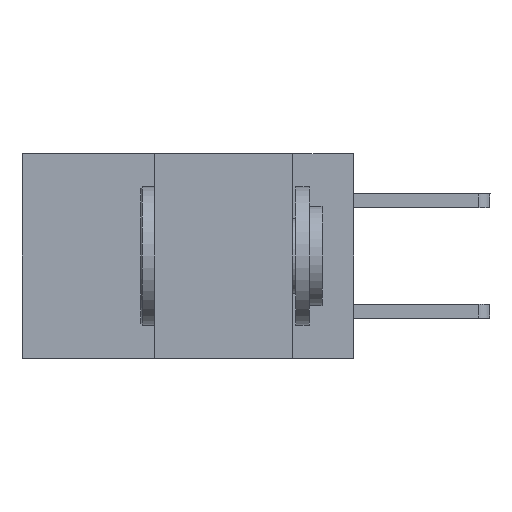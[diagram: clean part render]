
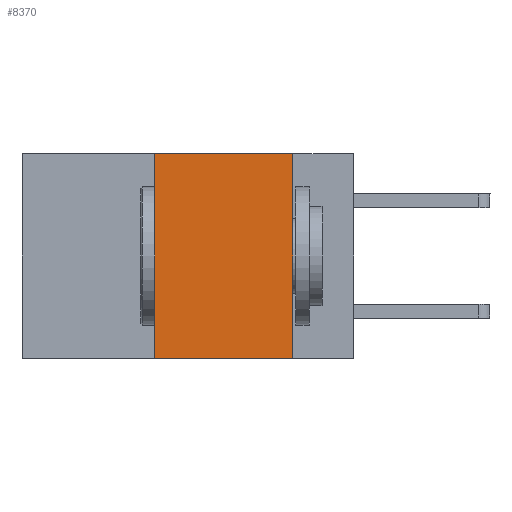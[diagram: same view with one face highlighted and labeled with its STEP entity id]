
A CAD part, left-side view. The second image highlights one B-rep face of the part: STEP entity #8370.
In plain terms, the highlighted planar face has unit normal (-1, 0, 0).
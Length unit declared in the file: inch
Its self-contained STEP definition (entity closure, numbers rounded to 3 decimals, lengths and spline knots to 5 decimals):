
#321 = VERTEX_POINT ( 'NONE', #10695 ) ;
#332 = EDGE_LOOP ( 'NONE', ( #8195, #7961, #2998, #5415 ) ) ;
#600 = VERTEX_POINT ( 'NONE', #6414 ) ;
#901 = CARTESIAN_POINT ( 'NONE',  ( 0., 0.36, -0.37 ) ) ;
#1046 = DIRECTION ( 'NONE',  ( 1., 0., 0. ) ) ;
#1924 = DIRECTION ( 'NONE',  ( 0., 0., 1. ) ) ;
#2919 = VERTEX_POINT ( 'NONE', #901 ) ;
#2998 = ORIENTED_EDGE ( 'NONE', *, *, #7019, .F. ) ;
#4089 = VERTEX_POINT ( 'NONE', #5334 ) ;
#4204 = LINE ( 'NONE', #5795, #11338 ) ;
#5086 = CARTESIAN_POINT ( 'NONE',  ( 0., 0.11, 0. ) ) ;
#5334 = CARTESIAN_POINT ( 'NONE',  ( 0., 0.36, 0. ) ) ;
#5415 = ORIENTED_EDGE ( 'NONE', *, *, #6902, .T. ) ;
#5714 = FACE_OUTER_BOUND ( 'NONE', #332, .T. ) ;
#5795 = CARTESIAN_POINT ( 'NONE',  ( 0., 0.6, 0. ) ) ;
#6414 = CARTESIAN_POINT ( 'NONE',  ( 0., 0.11, -0.37 ) ) ;
#6422 = VECTOR ( 'NONE', #1924, 39.37008 ) ;
#6792 = DIRECTION ( 'NONE',  ( 0., -1., 0. ) ) ;
#6895 = DIRECTION ( 'NONE',  ( 0., -1., 0. ) ) ;
#6902 = EDGE_CURVE ( 'NONE', #2919, #600, #7646, .T. ) ;
#7019 = EDGE_CURVE ( 'NONE', #2919, #4089, #11462, .T. ) ;
#7243 = PLANE ( 'NONE',  #10334 ) ;
#7646 = LINE ( 'NONE', #12556, #10190 ) ;
#7961 = ORIENTED_EDGE ( 'NONE', *, *, #10478, .F. ) ;
#8195 = ORIENTED_EDGE ( 'NONE', *, *, #12413, .F. ) ;
#8217 = DIRECTION ( 'NONE',  ( 0., 0., -1. ) ) ;
#8370 = ADVANCED_FACE ( 'NONE', ( #5714 ), #7243, .F. ) ;
#9118 = CARTESIAN_POINT ( 'NONE',  ( 0., 0.6, 0. ) ) ;
#10012 = VECTOR ( 'NONE', #10878, 39.37008 ) ;
#10190 = VECTOR ( 'NONE', #6895, 39.37008 ) ;
#10334 = AXIS2_PLACEMENT_3D ( 'NONE', #9118, #1046, #8217 ) ;
#10478 = EDGE_CURVE ( 'NONE', #4089, #321, #4204, .T. ) ;
#10695 = CARTESIAN_POINT ( 'NONE',  ( 0., 0.11, 0. ) ) ;
#10807 = CARTESIAN_POINT ( 'NONE',  ( 0., 0.36, 0. ) ) ;
#10878 = DIRECTION ( 'NONE',  ( 0., 0., -1. ) ) ;
#11338 = VECTOR ( 'NONE', #6792, 39.37008 ) ;
#11462 = LINE ( 'NONE', #10807, #6422 ) ;
#12413 = EDGE_CURVE ( 'NONE', #321, #600, #12453, .T. ) ;
#12453 = LINE ( 'NONE', #5086, #10012 ) ;
#12556 = CARTESIAN_POINT ( 'NONE',  ( 0., 0.6, -0.37 ) ) ;
